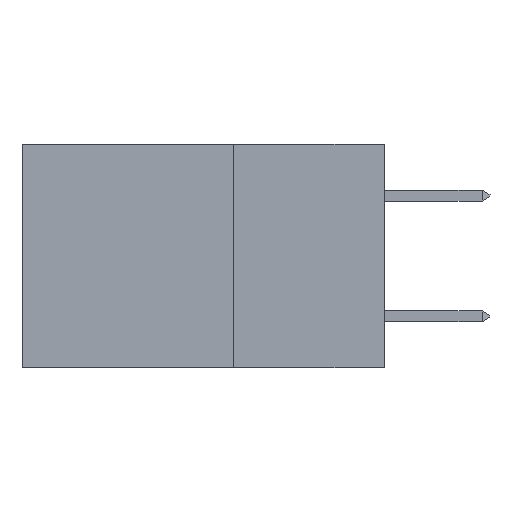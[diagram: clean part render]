
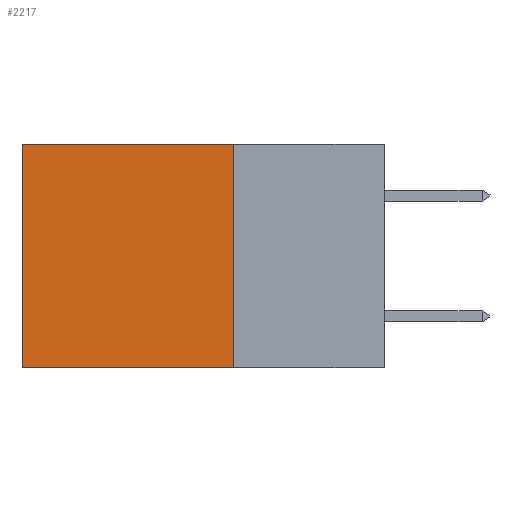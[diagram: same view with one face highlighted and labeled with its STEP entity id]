
A CAD part, left-side view. The second image highlights one B-rep face of the part: STEP entity #2217.
In plain terms, the highlighted planar face has unit normal (-1, 0, 0).
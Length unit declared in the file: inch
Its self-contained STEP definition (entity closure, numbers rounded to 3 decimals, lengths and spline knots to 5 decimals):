
#316 = CARTESIAN_POINT ( 'NONE',  ( 0.2875, 0.25, 0. ) ) ;
#1796 = LINE ( 'NONE', #11420, #10733 ) ;
#2022 = EDGE_LOOP ( 'NONE', ( #7654, #6583, #9765, #8594 ) ) ;
#2217 = ADVANCED_FACE ( 'NONE', ( #10697 ), #10707, .F. ) ;
#2647 = DIRECTION ( 'NONE',  ( 0., 1., 0. ) ) ;
#2871 = CARTESIAN_POINT ( 'NONE',  ( 0.2875, 0.25, -0.37 ) ) ;
#3246 = DIRECTION ( 'NONE',  ( 0., 0., -1. ) ) ;
#3801 = VERTEX_POINT ( 'NONE', #316 ) ;
#3984 = VERTEX_POINT ( 'NONE', #4317 ) ;
#4080 = CARTESIAN_POINT ( 'NONE',  ( 0.2875, 0.25, 0. ) ) ;
#4223 = VECTOR ( 'NONE', #2647, 39.37008 ) ;
#4317 = CARTESIAN_POINT ( 'NONE',  ( 0.2875, 0.6, -0.37 ) ) ;
#4540 = VECTOR ( 'NONE', #8244, 39.37008 ) ;
#5123 = CARTESIAN_POINT ( 'NONE',  ( 0.2875, 0.25, 0. ) ) ;
#5403 = EDGE_CURVE ( 'NONE', #3801, #7859, #9387, .T. ) ;
#5632 = CARTESIAN_POINT ( 'NONE',  ( 0.2875, 0.25, -0.37 ) ) ;
#6476 = CARTESIAN_POINT ( 'NONE',  ( 0.2875, 0.25, 0. ) ) ;
#6583 = ORIENTED_EDGE ( 'NONE', *, *, #10353, .F. ) ;
#7654 = ORIENTED_EDGE ( 'NONE', *, *, #7975, .T. ) ;
#7856 = CARTESIAN_POINT ( 'NONE',  ( 0.2875, 0.6, 0. ) ) ;
#7857 = DIRECTION ( 'NONE',  ( 1., 0., 0. ) ) ;
#7859 = VERTEX_POINT ( 'NONE', #5632 ) ;
#7975 = EDGE_CURVE ( 'NONE', #10909, #3984, #1796, .T. ) ;
#8042 = LINE ( 'NONE', #2871, #4223 ) ;
#8244 = DIRECTION ( 'NONE',  ( 0., 1., 0. ) ) ;
#8594 = ORIENTED_EDGE ( 'NONE', *, *, #10560, .T. ) ;
#9118 = AXIS2_PLACEMENT_3D ( 'NONE', #4080, #7857, #3246 ) ;
#9387 = LINE ( 'NONE', #5123, #9812 ) ;
#9765 = ORIENTED_EDGE ( 'NONE', *, *, #5403, .F. ) ;
#9812 = VECTOR ( 'NONE', #11718, 39.37008 ) ;
#10353 = EDGE_CURVE ( 'NONE', #7859, #3984, #8042, .T. ) ;
#10460 = DIRECTION ( 'NONE',  ( 0., 0., -1. ) ) ;
#10526 = LINE ( 'NONE', #6476, #4540 ) ;
#10560 = EDGE_CURVE ( 'NONE', #3801, #10909, #10526, .T. ) ;
#10697 = FACE_OUTER_BOUND ( 'NONE', #2022, .T. ) ;
#10707 = PLANE ( 'NONE',  #9118 ) ;
#10733 = VECTOR ( 'NONE', #10460, 39.37008 ) ;
#10909 = VERTEX_POINT ( 'NONE', #7856 ) ;
#11420 = CARTESIAN_POINT ( 'NONE',  ( 0.2875, 0.6, 0. ) ) ;
#11718 = DIRECTION ( 'NONE',  ( 0., 0., -1. ) ) ;
